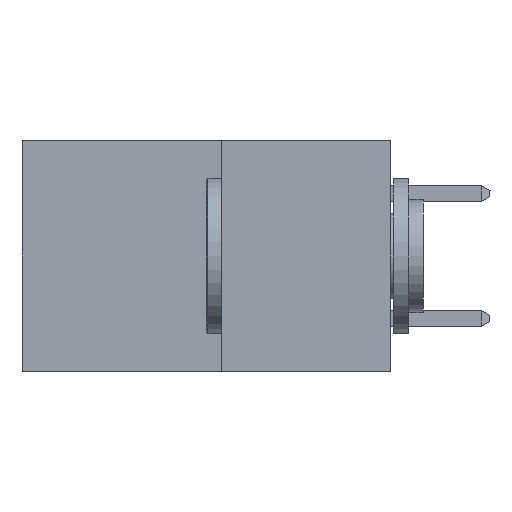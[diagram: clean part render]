
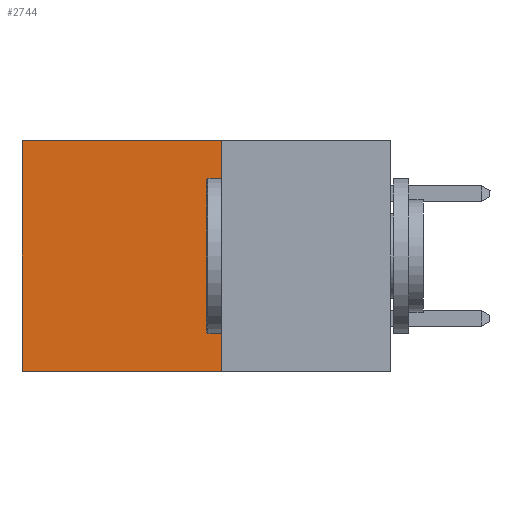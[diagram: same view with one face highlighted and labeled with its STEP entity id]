
A CAD part, left-side view. The second image highlights one B-rep face of the part: STEP entity #2744.
In plain terms, the highlighted planar face has unit normal (-1, 0, 0).
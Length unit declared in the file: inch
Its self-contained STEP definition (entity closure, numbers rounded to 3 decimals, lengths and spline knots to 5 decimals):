
#721 = VECTOR ( 'NONE', #5303, 39.37008 ) ;
#1021 = PLANE ( 'NONE',  #4602 ) ;
#1062 = EDGE_CURVE ( 'NONE', #2908, #7309, #6020, .T. ) ;
#2011 = CARTESIAN_POINT ( 'NONE',  ( 0.277, 0.27, -0.37 ) ) ;
#2421 = FACE_OUTER_BOUND ( 'NONE', #11318, .T. ) ;
#2551 = VERTEX_POINT ( 'NONE', #4599 ) ;
#2565 = EDGE_CURVE ( 'NONE', #12187, #2551, #7544, .T. ) ;
#2744 = ADVANCED_FACE ( 'NONE', ( #2421 ), #1021, .F. ) ;
#2745 = CARTESIAN_POINT ( 'NONE',  ( 0.277, 0.27, -0.37 ) ) ;
#2763 = DIRECTION ( 'NONE',  ( 0., 1., 0. ) ) ;
#2852 = ORIENTED_EDGE ( 'NONE', *, *, #2565, .F. ) ;
#2908 = VERTEX_POINT ( 'NONE', #10391 ) ;
#3192 = DIRECTION ( 'NONE',  ( 1., 0., 0. ) ) ;
#4248 = VECTOR ( 'NONE', #12441, 39.37008 ) ;
#4342 = VECTOR ( 'NONE', #2763, 39.37008 ) ;
#4423 = ORIENTED_EDGE ( 'NONE', *, *, #9635, .T. ) ;
#4599 = CARTESIAN_POINT ( 'NONE',  ( 0.277, 0.27, -0.37 ) ) ;
#4602 = AXIS2_PLACEMENT_3D ( 'NONE', #2011, #3192, #11509 ) ;
#5035 = CARTESIAN_POINT ( 'NONE',  ( 0.277, 0.59, -0.37 ) ) ;
#5303 = DIRECTION ( 'NONE',  ( 0., 0., -1. ) ) ;
#5697 = EDGE_CURVE ( 'NONE', #2551, #7309, #13421, .T. ) ;
#5903 = CARTESIAN_POINT ( 'NONE',  ( 0.277, 0.27, 0. ) ) ;
#6020 = LINE ( 'NONE', #9087, #721 ) ;
#6423 = DIRECTION ( 'NONE',  ( 0., 0., -1. ) ) ;
#6540 = CARTESIAN_POINT ( 'NONE',  ( 0.277, 0.27, -0.37 ) ) ;
#7309 = VERTEX_POINT ( 'NONE', #5035 ) ;
#7544 = LINE ( 'NONE', #6540, #12954 ) ;
#7671 = CARTESIAN_POINT ( 'NONE',  ( 0.277, 0.27, 0. ) ) ;
#9087 = CARTESIAN_POINT ( 'NONE',  ( 0.277, 0.59, -0.37 ) ) ;
#9602 = ORIENTED_EDGE ( 'NONE', *, *, #1062, .T. ) ;
#9635 = EDGE_CURVE ( 'NONE', #12187, #2908, #10279, .T. ) ;
#10279 = LINE ( 'NONE', #5903, #4248 ) ;
#10391 = CARTESIAN_POINT ( 'NONE',  ( 0.277, 0.59, 0. ) ) ;
#11318 = EDGE_LOOP ( 'NONE', ( #9602, #13155, #2852, #4423 ) ) ;
#11509 = DIRECTION ( 'NONE',  ( 0., 0., -1. ) ) ;
#12187 = VERTEX_POINT ( 'NONE', #7671 ) ;
#12441 = DIRECTION ( 'NONE',  ( 0., 1., 0. ) ) ;
#12954 = VECTOR ( 'NONE', #6423, 39.37008 ) ;
#13155 = ORIENTED_EDGE ( 'NONE', *, *, #5697, .F. ) ;
#13421 = LINE ( 'NONE', #2745, #4342 ) ;
